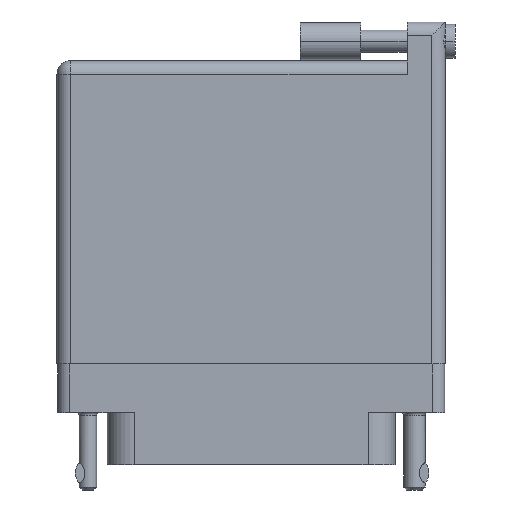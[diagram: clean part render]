
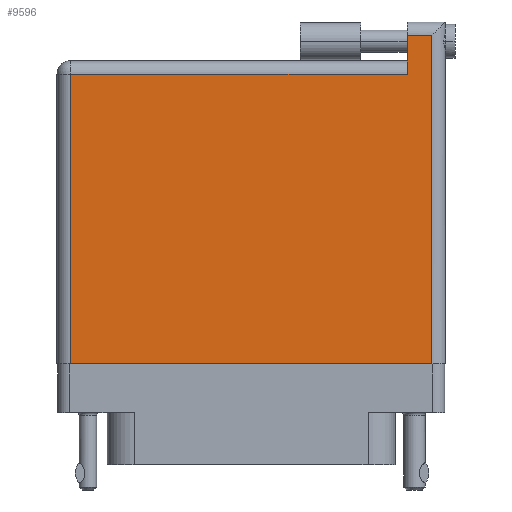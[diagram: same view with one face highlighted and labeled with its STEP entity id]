
A CAD part, front view. The second image highlights one B-rep face of the part: STEP entity #9596.
In plain terms, the highlighted face is planar.
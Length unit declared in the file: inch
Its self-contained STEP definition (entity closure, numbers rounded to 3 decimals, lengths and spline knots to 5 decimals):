
#1294 = VERTEX_POINT ( 'NONE', #37147 ) ;
#5245 = LINE ( 'NONE', #20842, #29849 ) ;
#5415 = ORIENTED_EDGE ( 'NONE', *, *, #8722, .T. ) ;
#6076 = VECTOR ( 'NONE', #11164, 39.37008 ) ;
#6532 = DIRECTION ( 'NONE',  ( -1., 0., 0. ) ) ;
#7834 = VECTOR ( 'NONE', #28900, 39.37008 ) ;
#8421 = EDGE_CURVE ( 'NONE', #33308, #32324, #5245, .T. ) ;
#8722 = EDGE_CURVE ( 'NONE', #40824, #38218, #45240, .T. ) ;
#9203 = VERTEX_POINT ( 'NONE', #14504 ) ;
#9596 = ADVANCED_FACE ( 'NONE', ( #36325 ), #31378, .F. ) ;
#9936 = EDGE_CURVE ( 'NONE', #38218, #9203, #36012, .T. ) ;
#10040 = DIRECTION ( 'NONE',  ( -1., 0., 0. ) ) ;
#10956 = CARTESIAN_POINT ( 'NONE',  ( 0.807, 1.396, 0.4495 ) ) ;
#11164 = DIRECTION ( 'NONE',  ( 0., -1., 0. ) ) ;
#11742 = ORIENTED_EDGE ( 'NONE', *, *, #15798, .T. ) ;
#14504 = CARTESIAN_POINT ( 'NONE',  ( 0.934, -0.1, 0.4495 ) ) ;
#15798 = EDGE_CURVE ( 'NONE', #1294, #33308, #39632, .T. ) ;
#16971 = EDGE_LOOP ( 'NONE', ( #20759, #44367, #11742, #31571, #31041, #5415 ) ) ;
#18001 = CARTESIAN_POINT ( 'NONE',  ( -1.004, 1.596, 0.4495 ) ) ;
#20232 = DIRECTION ( 'NONE',  ( -1., 0., 0. ) ) ;
#20367 = CARTESIAN_POINT ( 'NONE',  ( -1.004, -0.1, 0.4495 ) ) ;
#20612 = EDGE_CURVE ( 'NONE', #9203, #1294, #20697, .T. ) ;
#20697 = LINE ( 'NONE', #43337, #7834 ) ;
#20759 = ORIENTED_EDGE ( 'NONE', *, *, #9936, .T. ) ;
#20842 = CARTESIAN_POINT ( 'NONE',  ( 0.807, 1.666, 0.4495 ) ) ;
#26460 = EDGE_CURVE ( 'NONE', #32324, #40824, #35399, .T. ) ;
#28900 = DIRECTION ( 'NONE',  ( 0., 1., 0. ) ) ;
#29849 = VECTOR ( 'NONE', #35047, 39.37008 ) ;
#30664 = AXIS2_PLACEMENT_3D ( 'NONE', #39073, #33577, #6532 ) ;
#31041 = ORIENTED_EDGE ( 'NONE', *, *, #26460, .T. ) ;
#31378 = PLANE ( 'NONE',  #30664 ) ;
#31571 = ORIENTED_EDGE ( 'NONE', *, *, #8421, .T. ) ;
#31680 = CARTESIAN_POINT ( 'NONE',  ( -1.004, 1.396, 0.4495 ) ) ;
#32324 = VERTEX_POINT ( 'NONE', #10956 ) ;
#33308 = VERTEX_POINT ( 'NONE', #35819 ) ;
#33498 = VECTOR ( 'NONE', #10040, 39.37008 ) ;
#33577 = DIRECTION ( 'NONE',  ( 0., 0., -1. ) ) ;
#34179 = CARTESIAN_POINT ( 'NONE',  ( -0.934, 1.396, 0.4495 ) ) ;
#35047 = DIRECTION ( 'NONE',  ( 0., -1., 0. ) ) ;
#35052 = DIRECTION ( 'NONE',  ( 1., 0., 0. ) ) ;
#35399 = LINE ( 'NONE', #31680, #36401 ) ;
#35819 = CARTESIAN_POINT ( 'NONE',  ( 0.807, 1.596, 0.4495 ) ) ;
#36012 = LINE ( 'NONE', #20367, #47389 ) ;
#36325 = FACE_OUTER_BOUND ( 'NONE', #16971, .T. ) ;
#36401 = VECTOR ( 'NONE', #20232, 39.37008 ) ;
#37147 = CARTESIAN_POINT ( 'NONE',  ( 0.934, 1.596, 0.4495 ) ) ;
#38218 = VERTEX_POINT ( 'NONE', #40242 ) ;
#39073 = CARTESIAN_POINT ( 'NONE',  ( -1.004, 1.466, 0.4495 ) ) ;
#39632 = LINE ( 'NONE', #18001, #33498 ) ;
#40242 = CARTESIAN_POINT ( 'NONE',  ( -0.934, -0.1, 0.4495 ) ) ;
#40824 = VERTEX_POINT ( 'NONE', #34179 ) ;
#41990 = CARTESIAN_POINT ( 'NONE',  ( -0.934, -0.1, 0.4495 ) ) ;
#43337 = CARTESIAN_POINT ( 'NONE',  ( 0.934, 1.666, 0.4495 ) ) ;
#44367 = ORIENTED_EDGE ( 'NONE', *, *, #20612, .T. ) ;
#45240 = LINE ( 'NONE', #41990, #6076 ) ;
#47389 = VECTOR ( 'NONE', #35052, 39.37008 ) ;
